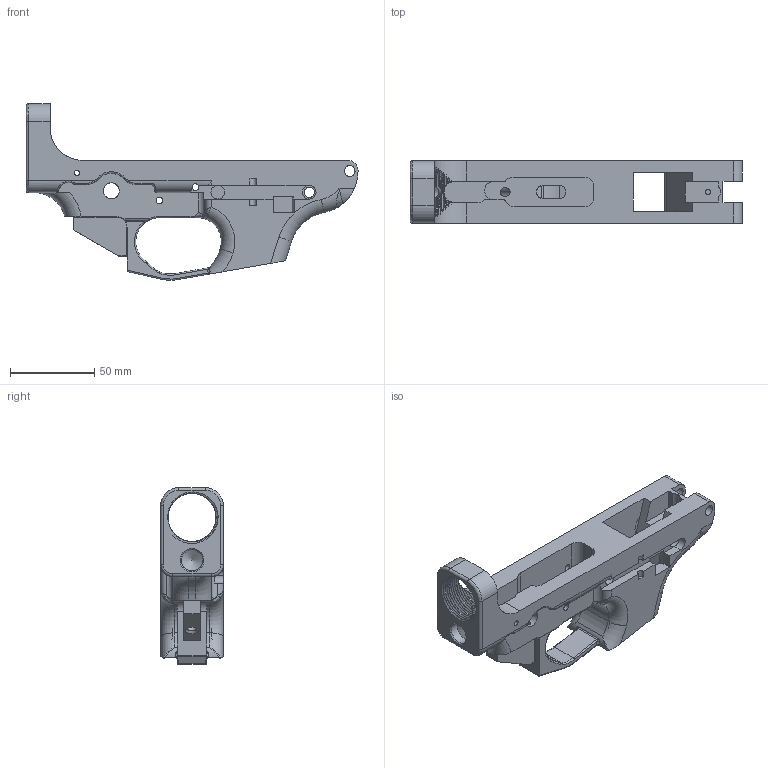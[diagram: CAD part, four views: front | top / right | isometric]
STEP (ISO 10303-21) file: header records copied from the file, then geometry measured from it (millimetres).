
FILE_DESCRIPTION (( 'STEP AP214' ), '1' );
FILE_NAME ('Gluty_V0.2A.STEP', '2016-02-15T23:17:00', ( 'WarFairy' ), ( '' ), 'SwSTEP 2.0', 'SolidWorks 2015', '' );
FILE_SCHEMA (( 'AUTOMOTIVE_DESIGN' ));
Length unit declared in the file: millimetre
Products named in the file (1): Gluty_V0.2A
Bounding box: 197.08 x 37.13 x 104.92 mm (x, y, z)
Volume: 167366.4 mm3; surface area: 56263.6 mm2
Topology: 1 solids, 1 shells, 349 faces, 994 edges, 624 vertices
Faces by surface type: cylinder 144, plane 87, bspline 71, torus 40, cone 5, sphere 2
Full cylindrical faces by diameter (mm): 3 x1, 3.175 x3, 3.969 x4, 5.105 x1, 6 x1, 6.375 x2, 6.477 x2, 8 x2, 9.525 x2, 12.7 x1, 16.2 x1
Entity records: 37922 total; most frequent: CARTESIAN_POINT 29720, ORIENTED_EDGE 1872, DIRECTION 1452, EDGE_CURVE 936, VERTEX_POINT 605, AXIS2_PLACEMENT_3D 553, EDGE_LOOP 401, FACE_OUTER_BOUND 369
